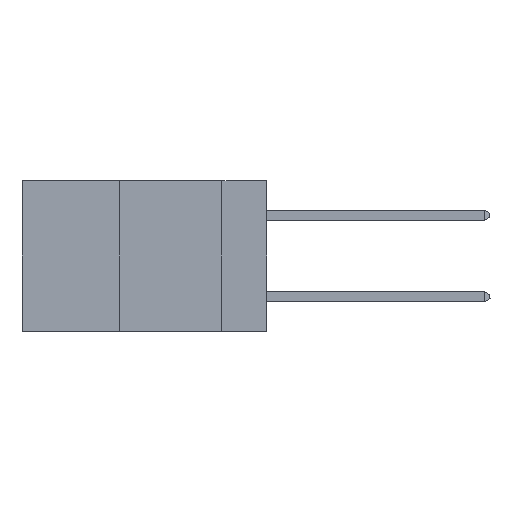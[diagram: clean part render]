
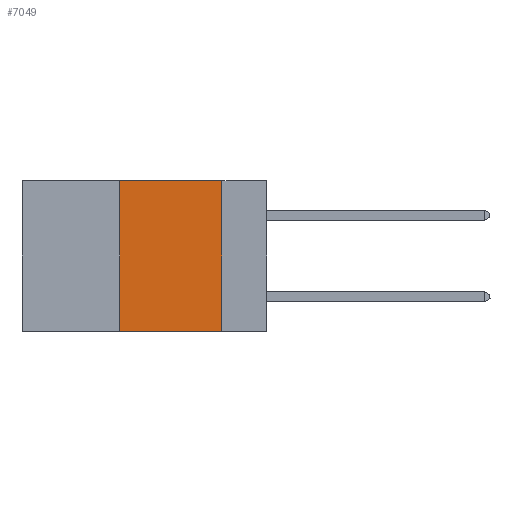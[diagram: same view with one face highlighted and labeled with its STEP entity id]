
A CAD part, left-side view. The second image highlights one B-rep face of the part: STEP entity #7049.
In plain terms, the highlighted planar face has unit normal (-1, 0, 0).
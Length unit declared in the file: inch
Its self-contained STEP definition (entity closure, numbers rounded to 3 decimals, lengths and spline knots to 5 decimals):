
#164 = CARTESIAN_POINT ( 'NONE',  ( 0., 0.11, 0. ) ) ;
#532 = ORIENTED_EDGE ( 'NONE', *, *, #10252, .F. ) ;
#536 = ORIENTED_EDGE ( 'NONE', *, *, #6013, .T. ) ;
#549 = ORIENTED_EDGE ( 'NONE', *, *, #12199, .F. ) ;
#813 = ORIENTED_EDGE ( 'NONE', *, *, #6097, .F. ) ;
#1143 = DIRECTION ( 'NONE',  ( 0., 0., -1. ) ) ;
#1715 = CARTESIAN_POINT ( 'NONE',  ( 0., 0.36, 0. ) ) ;
#2328 = CARTESIAN_POINT ( 'NONE',  ( 0., 0.6, 0. ) ) ;
#3302 = CARTESIAN_POINT ( 'NONE',  ( 0., 0.36, 0. ) ) ;
#3340 = VERTEX_POINT ( 'NONE', #164 ) ;
#3492 = DIRECTION ( 'NONE',  ( 0., -1., 0. ) ) ;
#4457 = PLANE ( 'NONE',  #7421 ) ;
#4866 = VERTEX_POINT ( 'NONE', #6089 ) ;
#5844 = FACE_OUTER_BOUND ( 'NONE', #8765, .T. ) ;
#6013 = EDGE_CURVE ( 'NONE', #4866, #7267, #6574, .T. ) ;
#6059 = VECTOR ( 'NONE', #9944, 39.37008 ) ;
#6089 = CARTESIAN_POINT ( 'NONE',  ( 0., 0.36, -0.37 ) ) ;
#6097 = EDGE_CURVE ( 'NONE', #3340, #7267, #13673, .T. ) ;
#6099 = LINE ( 'NONE', #2328, #14231 ) ;
#6211 = VECTOR ( 'NONE', #13536, 39.37008 ) ;
#6574 = LINE ( 'NONE', #13916, #6211 ) ;
#7049 = ADVANCED_FACE ( 'NONE', ( #5844 ), #4457, .F. ) ;
#7267 = VERTEX_POINT ( 'NONE', #10305 ) ;
#7421 = AXIS2_PLACEMENT_3D ( 'NONE', #9509, #9688, #1143 ) ;
#8141 = VECTOR ( 'NONE', #12487, 39.37008 ) ;
#8582 = VERTEX_POINT ( 'NONE', #1715 ) ;
#8765 = EDGE_LOOP ( 'NONE', ( #813, #532, #549, #536 ) ) ;
#9509 = CARTESIAN_POINT ( 'NONE',  ( 0., 0.6, 0. ) ) ;
#9688 = DIRECTION ( 'NONE',  ( 1., 0., 0. ) ) ;
#9944 = DIRECTION ( 'NONE',  ( 0., 0., 1. ) ) ;
#10252 = EDGE_CURVE ( 'NONE', #8582, #3340, #6099, .T. ) ;
#10305 = CARTESIAN_POINT ( 'NONE',  ( 0., 0.11, -0.37 ) ) ;
#11992 = CARTESIAN_POINT ( 'NONE',  ( 0., 0.11, 0. ) ) ;
#12132 = LINE ( 'NONE', #3302, #6059 ) ;
#12199 = EDGE_CURVE ( 'NONE', #4866, #8582, #12132, .T. ) ;
#12487 = DIRECTION ( 'NONE',  ( 0., 0., -1. ) ) ;
#13536 = DIRECTION ( 'NONE',  ( 0., -1., 0. ) ) ;
#13673 = LINE ( 'NONE', #11992, #8141 ) ;
#13916 = CARTESIAN_POINT ( 'NONE',  ( 0., 0.6, -0.37 ) ) ;
#14231 = VECTOR ( 'NONE', #3492, 39.37008 ) ;
